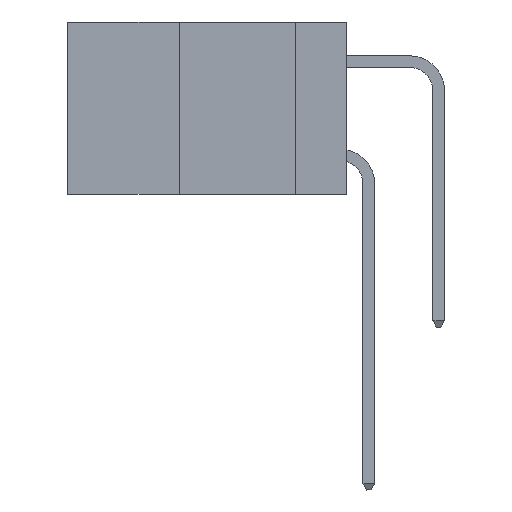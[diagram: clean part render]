
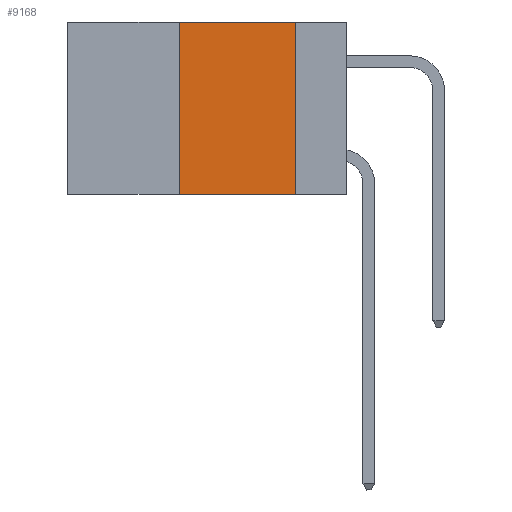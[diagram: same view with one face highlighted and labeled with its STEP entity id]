
A CAD part, left-side view. The second image highlights one B-rep face of the part: STEP entity #9168.
In plain terms, the highlighted planar face has unit normal (-1, 0, 0).
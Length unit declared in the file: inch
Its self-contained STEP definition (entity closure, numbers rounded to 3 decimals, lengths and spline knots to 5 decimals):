
#1998 = EDGE_CURVE ( 'NONE', #28051, #32907, #40540, .T. ) ;
#2691 = LINE ( 'NONE', #27074, #18181 ) ;
#5228 = EDGE_CURVE ( 'NONE', #28051, #23270, #2691, .T. ) ;
#6290 = EDGE_LOOP ( 'NONE', ( #7990, #18755, #33076, #11718 ) ) ;
#7990 = ORIENTED_EDGE ( 'NONE', *, *, #8767, .F. ) ;
#8653 = CARTESIAN_POINT ( 'NONE',  ( 0., 0.11, 0. ) ) ;
#8767 = EDGE_CURVE ( 'NONE', #42306, #23270, #20962, .T. ) ;
#9168 = ADVANCED_FACE ( 'NONE', ( #26357 ), #27876, .F. ) ;
#10033 = CARTESIAN_POINT ( 'NONE',  ( 0., 0.11, -0.37 ) ) ;
#11718 = ORIENTED_EDGE ( 'NONE', *, *, #5228, .T. ) ;
#12202 = VECTOR ( 'NONE', #28350, 39.37008 ) ;
#12614 = LINE ( 'NONE', #18366, #13652 ) ;
#13652 = VECTOR ( 'NONE', #27963, 39.37008 ) ;
#15525 = DIRECTION ( 'NONE',  ( 1., 0., 0. ) ) ;
#17038 = DIRECTION ( 'NONE',  ( 0., -1., 0. ) ) ;
#18181 = VECTOR ( 'NONE', #17038, 39.37008 ) ;
#18366 = CARTESIAN_POINT ( 'NONE',  ( 0., 0.6, 0. ) ) ;
#18755 = ORIENTED_EDGE ( 'NONE', *, *, #40207, .F. ) ;
#20962 = LINE ( 'NONE', #8653, #12202 ) ;
#23270 = VERTEX_POINT ( 'NONE', #10033 ) ;
#26357 = FACE_OUTER_BOUND ( 'NONE', #6290, .T. ) ;
#27074 = CARTESIAN_POINT ( 'NONE',  ( 0., 0.6, -0.37 ) ) ;
#27876 = PLANE ( 'NONE',  #35594 ) ;
#27963 = DIRECTION ( 'NONE',  ( 0., -1., 0. ) ) ;
#28051 = VERTEX_POINT ( 'NONE', #38968 ) ;
#28350 = DIRECTION ( 'NONE',  ( 0., 0., -1. ) ) ;
#28580 = DIRECTION ( 'NONE',  ( 0., 0., -1. ) ) ;
#32907 = VERTEX_POINT ( 'NONE', #39612 ) ;
#33076 = ORIENTED_EDGE ( 'NONE', *, *, #1998, .F. ) ;
#33355 = CARTESIAN_POINT ( 'NONE',  ( 0., 0.11, 0. ) ) ;
#33622 = CARTESIAN_POINT ( 'NONE',  ( 0., 0.36, 0. ) ) ;
#34200 = CARTESIAN_POINT ( 'NONE',  ( 0., 0.6, 0. ) ) ;
#35594 = AXIS2_PLACEMENT_3D ( 'NONE', #34200, #15525, #28580 ) ;
#38968 = CARTESIAN_POINT ( 'NONE',  ( 0., 0.36, -0.37 ) ) ;
#39612 = CARTESIAN_POINT ( 'NONE',  ( 0., 0.36, 0. ) ) ;
#39904 = DIRECTION ( 'NONE',  ( 0., 0., 1. ) ) ;
#40207 = EDGE_CURVE ( 'NONE', #32907, #42306, #12614, .T. ) ;
#40540 = LINE ( 'NONE', #33622, #41575 ) ;
#41575 = VECTOR ( 'NONE', #39904, 39.37008 ) ;
#42306 = VERTEX_POINT ( 'NONE', #33355 ) ;
